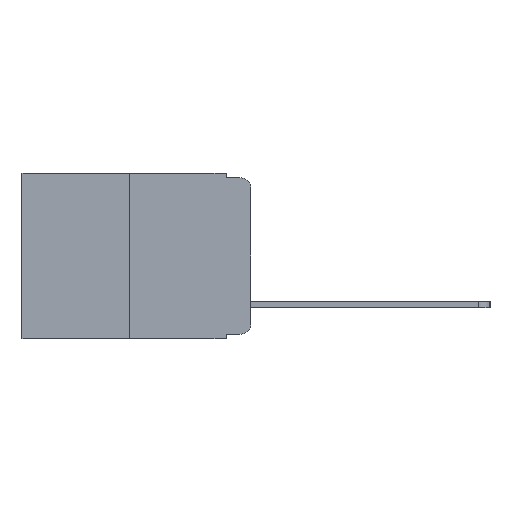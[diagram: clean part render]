
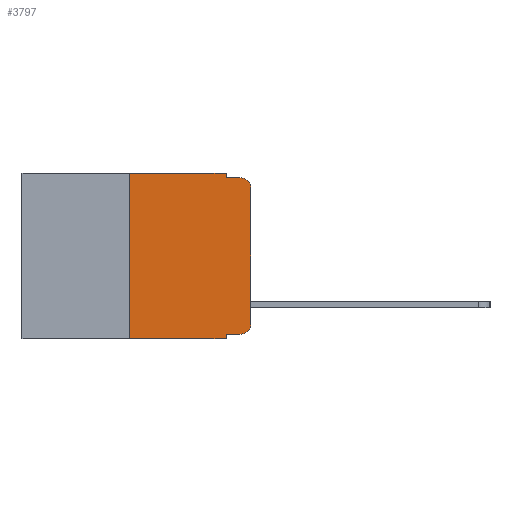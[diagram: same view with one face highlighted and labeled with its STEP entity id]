
A CAD part, left-side view. The second image highlights one B-rep face of the part: STEP entity #3797.
In plain terms, the highlighted planar face has unit normal (-1, 0, 0).
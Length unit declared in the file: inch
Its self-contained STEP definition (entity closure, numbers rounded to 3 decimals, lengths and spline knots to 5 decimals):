
#46 = AXIS2_PLACEMENT_3D ( 'NONE', #10140, #3880, #11143 ) ;
#493 = LINE ( 'NONE', #6136, #11596 ) ;
#663 = DIRECTION ( 'NONE',  ( 0., 0., 1. ) ) ;
#699 = CARTESIAN_POINT ( 'NONE',  ( 0., 0.02, -0.01 ) ) ;
#958 = VECTOR ( 'NONE', #663, 39.37008 ) ;
#1042 = CARTESIAN_POINT ( 'NONE',  ( 0., 0.02, -0.333 ) ) ;
#1164 = CARTESIAN_POINT ( 'NONE',  ( 0., 0.25, 0. ) ) ;
#1409 = ORIENTED_EDGE ( 'NONE', *, *, #5156, .F. ) ;
#1830 = EDGE_CURVE ( 'NONE', #6386, #7669, #12527, .T. ) ;
#2054 = EDGE_CURVE ( 'NONE', #8724, #9444, #7066, .T. ) ;
#2060 = CARTESIAN_POINT ( 'NONE',  ( 0., 0.02, -0.03 ) ) ;
#2232 = AXIS2_PLACEMENT_3D ( 'NONE', #2060, #9544, #3229 ) ;
#2285 = CARTESIAN_POINT ( 'NONE',  ( 0., 0.25, -0.343 ) ) ;
#2290 = VERTEX_POINT ( 'NONE', #6068 ) ;
#2416 = AXIS2_PLACEMENT_3D ( 'NONE', #3363, #12392, #12191 ) ;
#2934 = CARTESIAN_POINT ( 'NONE',  ( 0., 0.25, 0. ) ) ;
#3229 = DIRECTION ( 'NONE',  ( 0., 0., -1. ) ) ;
#3341 = CARTESIAN_POINT ( 'NONE',  ( 0., 0., -0.313 ) ) ;
#3363 = CARTESIAN_POINT ( 'NONE',  ( 0., 0.02, -0.313 ) ) ;
#3496 = FACE_OUTER_BOUND ( 'NONE', #11401, .T. ) ;
#3693 = VERTEX_POINT ( 'NONE', #6827 ) ;
#3797 = ADVANCED_FACE ( 'NONE', ( #3496 ), #12052, .F. ) ;
#3880 = DIRECTION ( 'NONE',  ( 1., 0., 0. ) ) ;
#4026 = EDGE_CURVE ( 'NONE', #2290, #8382, #7194, .T. ) ;
#4036 = CARTESIAN_POINT ( 'NONE',  ( 0., 0.051, 0. ) ) ;
#4112 = ORIENTED_EDGE ( 'NONE', *, *, #4473, .F. ) ;
#4172 = LINE ( 'NONE', #7250, #11728 ) ;
#4473 = EDGE_CURVE ( 'NONE', #9129, #9455, #493, .T. ) ;
#4989 = ORIENTED_EDGE ( 'NONE', *, *, #7323, .T. ) ;
#5156 = EDGE_CURVE ( 'NONE', #7669, #9129, #4172, .T. ) ;
#5545 = EDGE_CURVE ( 'NONE', #9455, #8382, #11716, .T. ) ;
#6004 = DIRECTION ( 'NONE',  ( 0., -1., 0. ) ) ;
#6068 = CARTESIAN_POINT ( 'NONE',  ( 0., 0., -0.03 ) ) ;
#6136 = CARTESIAN_POINT ( 'NONE',  ( 0., 0.051, 0. ) ) ;
#6183 = DIRECTION ( 'NONE',  ( 0., 0., -1. ) ) ;
#6386 = VERTEX_POINT ( 'NONE', #2285 ) ;
#6827 = CARTESIAN_POINT ( 'NONE',  ( 0., 0.051, -0.343 ) ) ;
#7066 = CIRCLE ( 'NONE', #2416, 0.02 ) ;
#7194 = CIRCLE ( 'NONE', #2232, 0.02 ) ;
#7250 = CARTESIAN_POINT ( 'NONE',  ( 0., 0.473, 0. ) ) ;
#7323 = EDGE_CURVE ( 'NONE', #9444, #2290, #12964, .T. ) ;
#7647 = EDGE_CURVE ( 'NONE', #9055, #3693, #12552, .T. ) ;
#7660 = CARTESIAN_POINT ( 'NONE',  ( 0., 0.051, -0.01 ) ) ;
#7669 = VERTEX_POINT ( 'NONE', #2934 ) ;
#7753 = VECTOR ( 'NONE', #13499, 39.37008 ) ;
#7778 = VECTOR ( 'NONE', #8971, 39.37008 ) ;
#7840 = LINE ( 'NONE', #10083, #10205 ) ;
#7965 = CARTESIAN_POINT ( 'NONE',  ( 0., 0.051, -0.333 ) ) ;
#8078 = CARTESIAN_POINT ( 'NONE',  ( 0., 0.051, -0.01 ) ) ;
#8261 = ORIENTED_EDGE ( 'NONE', *, *, #10250, .T. ) ;
#8382 = VERTEX_POINT ( 'NONE', #699 ) ;
#8724 = VERTEX_POINT ( 'NONE', #1042 ) ;
#8971 = DIRECTION ( 'NONE',  ( 0., -1., 0. ) ) ;
#9055 = VERTEX_POINT ( 'NONE', #9179 ) ;
#9082 = VECTOR ( 'NONE', #12050, 39.37008 ) ;
#9129 = VERTEX_POINT ( 'NONE', #4036 ) ;
#9179 = CARTESIAN_POINT ( 'NONE',  ( 0., 0.051, -0.333 ) ) ;
#9208 = ORIENTED_EDGE ( 'NONE', *, *, #12910, .T. ) ;
#9444 = VERTEX_POINT ( 'NONE', #3341 ) ;
#9455 = VERTEX_POINT ( 'NONE', #7660 ) ;
#9544 = DIRECTION ( 'NONE',  ( -1., 0., 0. ) ) ;
#9648 = VECTOR ( 'NONE', #10303, 39.37008 ) ;
#10083 = CARTESIAN_POINT ( 'NONE',  ( 0., 0.473, -0.343 ) ) ;
#10140 = CARTESIAN_POINT ( 'NONE',  ( 0., 0.473, 0. ) ) ;
#10205 = VECTOR ( 'NONE', #6004, 39.37008 ) ;
#10250 = EDGE_CURVE ( 'NONE', #6386, #3693, #7840, .T. ) ;
#10303 = DIRECTION ( 'NONE',  ( 0., 0., -1. ) ) ;
#10607 = ORIENTED_EDGE ( 'NONE', *, *, #1830, .F. ) ;
#10759 = ORIENTED_EDGE ( 'NONE', *, *, #4026, .T. ) ;
#11071 = ORIENTED_EDGE ( 'NONE', *, *, #5545, .F. ) ;
#11143 = DIRECTION ( 'NONE',  ( 0., 0., -1. ) ) ;
#11304 = CARTESIAN_POINT ( 'NONE',  ( 0., 0.051, 0. ) ) ;
#11401 = EDGE_LOOP ( 'NONE', ( #4989, #10759, #11071, #4112, #1409, #10607, #8261, #11540, #9208, #12126 ) ) ;
#11540 = ORIENTED_EDGE ( 'NONE', *, *, #7647, .F. ) ;
#11596 = VECTOR ( 'NONE', #6183, 39.37008 ) ;
#11640 = CARTESIAN_POINT ( 'NONE',  ( 0., 0., 0. ) ) ;
#11716 = LINE ( 'NONE', #8078, #9082 ) ;
#11728 = VECTOR ( 'NONE', #13154, 39.37008 ) ;
#12050 = DIRECTION ( 'NONE',  ( 0., -1., 0. ) ) ;
#12052 = PLANE ( 'NONE',  #46 ) ;
#12126 = ORIENTED_EDGE ( 'NONE', *, *, #2054, .T. ) ;
#12191 = DIRECTION ( 'NONE',  ( 0., 0., -1. ) ) ;
#12392 = DIRECTION ( 'NONE',  ( -1., 0., 0. ) ) ;
#12527 = LINE ( 'NONE', #1164, #958 ) ;
#12552 = LINE ( 'NONE', #11304, #9648 ) ;
#12910 = EDGE_CURVE ( 'NONE', #9055, #8724, #12985, .T. ) ;
#12964 = LINE ( 'NONE', #11640, #7753 ) ;
#12985 = LINE ( 'NONE', #7965, #7778 ) ;
#13154 = DIRECTION ( 'NONE',  ( 0., -1., 0. ) ) ;
#13499 = DIRECTION ( 'NONE',  ( 0., 0., 1. ) ) ;
